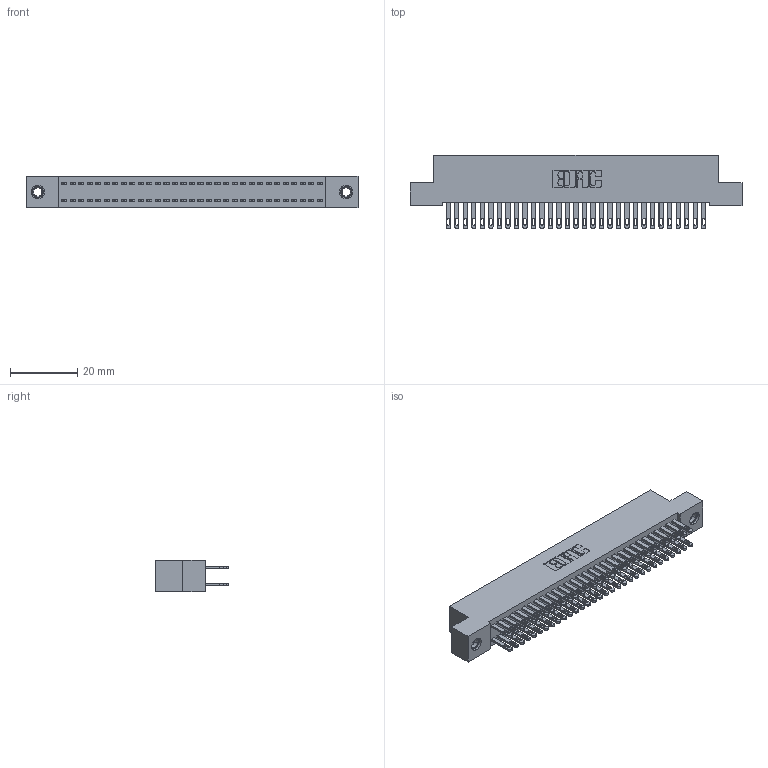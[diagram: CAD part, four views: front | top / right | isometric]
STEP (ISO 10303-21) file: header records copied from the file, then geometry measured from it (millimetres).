
FILE_DESCRIPTION (( 'STEP AP203' ), '1' );
FILE_NAME ('342-062-500-207.STEP', '2019-10-03T13:41:56', ( '' ), ( '' ), 'SwSTEP 2.0', 'SolidWorks 2016', '' );
FILE_SCHEMA (( 'CONFIG_CONTROL_DESIGN' ));
Length unit declared in the file: inch
Products named in the file (4): 342 Part_TI; 345-292-001_345-293-100; 345-250-001_345-250-005-103; 342-062-500-207
Assembly tree (65 placements, depth 2):
  342-062-500-207
    342 Part_TI
    345-292-001_345-293-100  x62
    345-250-001_345-250-005-103  x2
Bounding box: 99.06 x 21.85 x 9.4 mm (x, y, z)
Volume: 9025.2 mm3; surface area: 15039.2 mm2
Topology: 65 solids, 65 shells, 3146 faces, 9549 edges, 6358 vertices
Faces by surface type: plane 1958, cylinder 1172, cone 12, torus 4
Entity records: 22350 total; most frequent: CARTESIAN_POINT 3697, ORIENTED_EDGE 3626, DIRECTION 3211, EDGE_CURVE 1813, VECTOR 1661, LINE 1661, VERTEX_POINT 1204, AXIS2_PLACEMENT_3D 775
